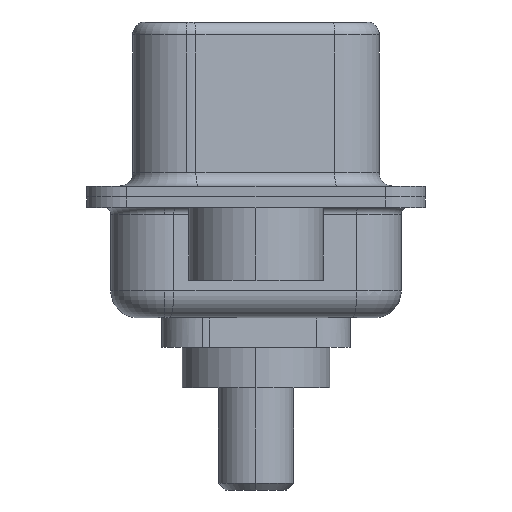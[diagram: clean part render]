
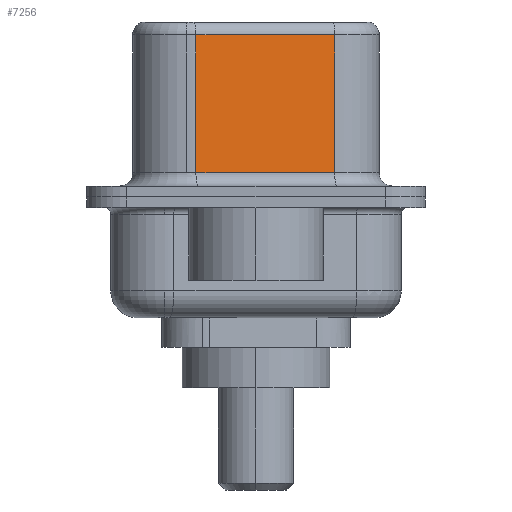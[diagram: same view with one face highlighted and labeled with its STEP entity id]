
A CAD part, left-side view. The second image highlights one B-rep face of the part: STEP entity #7256.
In plain terms, the highlighted planar face has unit normal (-0.985, -0.174, 0).
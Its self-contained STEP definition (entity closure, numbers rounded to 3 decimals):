
#327 = VERTEX_POINT ( 'NONE', #2947 ) ;
#1550 = VECTOR ( 'NONE', #7519, 1000. ) ;
#2112 = EDGE_LOOP ( 'NONE', ( #11105, #7538, #14677, #9319 ) ) ;
#2331 = CARTESIAN_POINT ( 'NONE',  ( 4.565, -2.927, 6.02 ) ) ;
#2560 = DIRECTION ( 'NONE',  ( 0., 0., -1. ) ) ;
#2714 = LINE ( 'NONE', #15365, #5880 ) ;
#2745 = CARTESIAN_POINT ( 'NONE',  ( 4.565, -2.927, 0.9 ) ) ;
#2947 = CARTESIAN_POINT ( 'NONE',  ( 3.655, 2.233, 0.9 ) ) ;
#3102 = FACE_OUTER_BOUND ( 'NONE', #2112, .T. ) ;
#3411 = LINE ( 'NONE', #2331, #12187 ) ;
#3485 = VECTOR ( 'NONE', #8467, 1000. ) ;
#3760 = EDGE_CURVE ( 'NONE', #5101, #327, #2714, .T. ) ;
#4402 = CARTESIAN_POINT ( 'NONE',  ( 4.565, -2.927, 0.9 ) ) ;
#5101 = VERTEX_POINT ( 'NONE', #15454 ) ;
#5512 = VERTEX_POINT ( 'NONE', #14944 ) ;
#5765 = EDGE_CURVE ( 'NONE', #5512, #10955, #13034, .T. ) ;
#5880 = VECTOR ( 'NONE', #2560, 1000. ) ;
#6280 = DIRECTION ( 'NONE',  ( 0.985, 0.174, 0. ) ) ;
#7256 = ADVANCED_FACE ( 'NONE', ( #3102 ), #13479, .F. ) ;
#7272 = CARTESIAN_POINT ( 'NONE',  ( 4.565, -2.927, 6.52 ) ) ;
#7519 = DIRECTION ( 'NONE',  ( 0.174, -0.985, 0. ) ) ;
#7538 = ORIENTED_EDGE ( 'NONE', *, *, #15603, .T. ) ;
#8317 = LINE ( 'NONE', #2745, #1550 ) ;
#8467 = DIRECTION ( 'NONE',  ( 0., 0., -1. ) ) ;
#8890 = EDGE_CURVE ( 'NONE', #327, #10955, #8317, .T. ) ;
#9319 = ORIENTED_EDGE ( 'NONE', *, *, #8890, .T. ) ;
#10955 = VERTEX_POINT ( 'NONE', #4402 ) ;
#11105 = ORIENTED_EDGE ( 'NONE', *, *, #5765, .F. ) ;
#11918 = DIRECTION ( 'NONE',  ( -0.174, 0.985, 0. ) ) ;
#12173 = AXIS2_PLACEMENT_3D ( 'NONE', #14645, #6280, #14693 ) ;
#12187 = VECTOR ( 'NONE', #11918, 1000. ) ;
#13034 = LINE ( 'NONE', #7272, #3485 ) ;
#13479 = PLANE ( 'NONE',  #12173 ) ;
#14645 = CARTESIAN_POINT ( 'NONE',  ( 4.565, -2.927, 6.52 ) ) ;
#14677 = ORIENTED_EDGE ( 'NONE', *, *, #3760, .T. ) ;
#14693 = DIRECTION ( 'NONE',  ( -0.174, 0.985, 0. ) ) ;
#14944 = CARTESIAN_POINT ( 'NONE',  ( 4.565, -2.927, 6.02 ) ) ;
#15365 = CARTESIAN_POINT ( 'NONE',  ( 3.655, 2.233, 6.52 ) ) ;
#15454 = CARTESIAN_POINT ( 'NONE',  ( 3.655, 2.233, 6.02 ) ) ;
#15603 = EDGE_CURVE ( 'NONE', #5512, #5101, #3411, .T. ) ;
